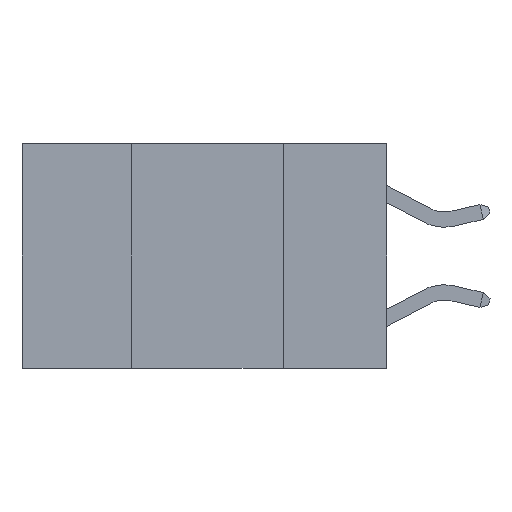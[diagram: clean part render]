
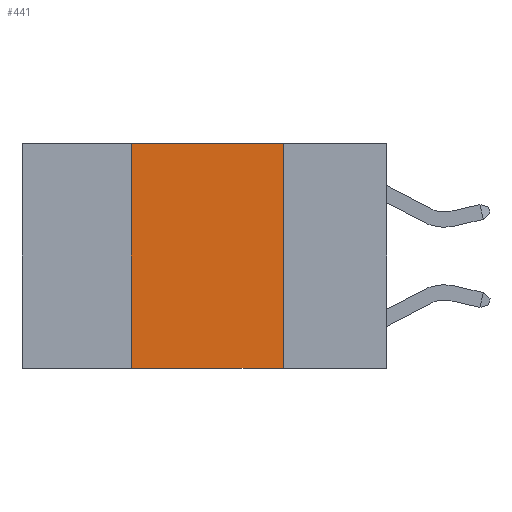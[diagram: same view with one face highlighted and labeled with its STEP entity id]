
A CAD part, left-side view. The second image highlights one B-rep face of the part: STEP entity #441.
In plain terms, the highlighted planar face has unit normal (-1, 0, 0).
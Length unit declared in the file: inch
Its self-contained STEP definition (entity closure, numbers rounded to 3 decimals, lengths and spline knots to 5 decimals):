
#177 = CARTESIAN_POINT ( 'NONE',  ( 0., 0.6, 0. ) ) ;
#441 = ADVANCED_FACE ( 'NONE', ( #11183 ), #12410, .F. ) ;
#616 = CARTESIAN_POINT ( 'NONE',  ( 0., 0.42, 0. ) ) ;
#1011 = EDGE_CURVE ( 'NONE', #4528, #10634, #1836, .T. ) ;
#1106 = LINE ( 'NONE', #10209, #5727 ) ;
#1539 = LINE ( 'NONE', #616, #9378 ) ;
#1698 = DIRECTION ( 'NONE',  ( 0., 0., -1. ) ) ;
#1836 = LINE ( 'NONE', #11280, #9362 ) ;
#2672 = CARTESIAN_POINT ( 'NONE',  ( 0., 0.42, 0. ) ) ;
#3066 = ORIENTED_EDGE ( 'NONE', *, *, #6314, .F. ) ;
#3362 = VERTEX_POINT ( 'NONE', #4194 ) ;
#4194 = CARTESIAN_POINT ( 'NONE',  ( 0., 0.42, -0.37 ) ) ;
#4528 = VERTEX_POINT ( 'NONE', #2672 ) ;
#4640 = DIRECTION ( 'NONE',  ( 0., -1., 0. ) ) ;
#4996 = VECTOR ( 'NONE', #8715, 39.37008 ) ;
#5727 = VECTOR ( 'NONE', #7337, 39.37008 ) ;
#6314 = EDGE_CURVE ( 'NONE', #10634, #9265, #1106, .T. ) ;
#6408 = AXIS2_PLACEMENT_3D ( 'NONE', #177, #12030, #1698 ) ;
#7337 = DIRECTION ( 'NONE',  ( 0., 0., -1. ) ) ;
#7505 = DIRECTION ( 'NONE',  ( 0., 0., 1. ) ) ;
#7625 = LINE ( 'NONE', #11560, #4996 ) ;
#7930 = CARTESIAN_POINT ( 'NONE',  ( 0., 0.17, -0.37 ) ) ;
#7957 = ORIENTED_EDGE ( 'NONE', *, *, #11268, .F. ) ;
#8715 = DIRECTION ( 'NONE',  ( 0., -1., 0. ) ) ;
#8719 = ORIENTED_EDGE ( 'NONE', *, *, #1011, .F. ) ;
#9157 = EDGE_CURVE ( 'NONE', #3362, #9265, #7625, .T. ) ;
#9265 = VERTEX_POINT ( 'NONE', #7930 ) ;
#9362 = VECTOR ( 'NONE', #4640, 39.37008 ) ;
#9378 = VECTOR ( 'NONE', #7505, 39.37008 ) ;
#9479 = CARTESIAN_POINT ( 'NONE',  ( 0., 0.17, 0. ) ) ;
#10209 = CARTESIAN_POINT ( 'NONE',  ( 0., 0.17, 0. ) ) ;
#10634 = VERTEX_POINT ( 'NONE', #9479 ) ;
#11110 = ORIENTED_EDGE ( 'NONE', *, *, #9157, .T. ) ;
#11183 = FACE_OUTER_BOUND ( 'NONE', #11808, .T. ) ;
#11268 = EDGE_CURVE ( 'NONE', #3362, #4528, #1539, .T. ) ;
#11280 = CARTESIAN_POINT ( 'NONE',  ( 0., 0.6, 0. ) ) ;
#11560 = CARTESIAN_POINT ( 'NONE',  ( 0., 0.6, -0.37 ) ) ;
#11808 = EDGE_LOOP ( 'NONE', ( #3066, #8719, #7957, #11110 ) ) ;
#12030 = DIRECTION ( 'NONE',  ( 1., 0., 0. ) ) ;
#12410 = PLANE ( 'NONE',  #6408 ) ;
